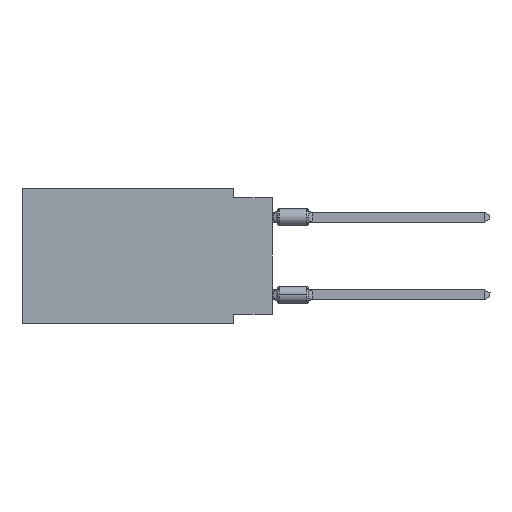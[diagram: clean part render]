
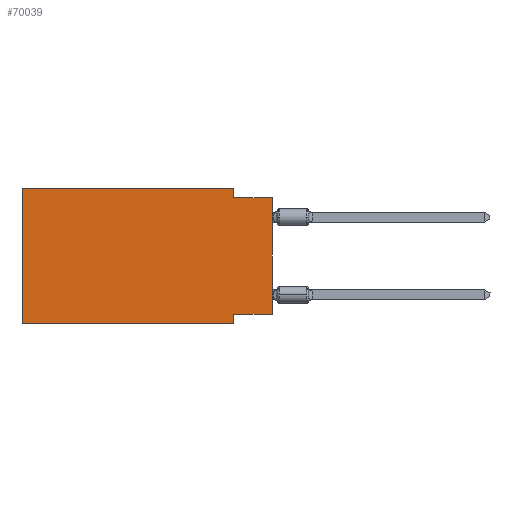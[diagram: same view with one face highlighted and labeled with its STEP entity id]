
A CAD part, left-side view. The second image highlights one B-rep face of the part: STEP entity #70039.
In plain terms, the highlighted planar face has unit normal (-1, 0, 0).
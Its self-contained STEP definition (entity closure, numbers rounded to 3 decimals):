
#1227 = ORIENTED_EDGE ( 'NONE', *, *, #39790, .F. ) ;
#2309 = EDGE_LOOP ( 'NONE', ( #7311, #1227, #25626, #28948, #22406, #39663, #37790, #55043 ) ) ;
#2848 = DIRECTION ( 'NONE',  ( 0., 0., -1. ) ) ;
#3873 = CARTESIAN_POINT ( 'NONE',  ( 0., 16.383, 0. ) ) ;
#4240 = CARTESIAN_POINT ( 'NONE',  ( 0., 16.383, 0. ) ) ;
#4320 = CARTESIAN_POINT ( 'NONE',  ( 0., 2.54, -8.255 ) ) ;
#4486 = VERTEX_POINT ( 'NONE', #47681 ) ;
#7311 = ORIENTED_EDGE ( 'NONE', *, *, #52793, .T. ) ;
#8600 = DIRECTION ( 'NONE',  ( 0., 0., -1. ) ) ;
#12248 = VERTEX_POINT ( 'NONE', #57876 ) ;
#12570 = EDGE_CURVE ( 'NONE', #12248, #4486, #19305, .T. ) ;
#13550 = AXIS2_PLACEMENT_3D ( 'NONE', #3873, #14925, #25629 ) ;
#14925 = DIRECTION ( 'NONE',  ( 1., 0., 0. ) ) ;
#16341 = CARTESIAN_POINT ( 'NONE',  ( 0., 16.383, -8.89 ) ) ;
#18256 = CARTESIAN_POINT ( 'NONE',  ( 0., 2.54, 0. ) ) ;
#19305 = LINE ( 'NONE', #18256, #48768 ) ;
#20276 = VECTOR ( 'NONE', #40275, 1000. ) ;
#22406 = ORIENTED_EDGE ( 'NONE', *, *, #34419, .F. ) ;
#23766 = EDGE_CURVE ( 'NONE', #64450, #54979, #24576, .T. ) ;
#24576 = LINE ( 'NONE', #68429, #20276 ) ;
#25626 = ORIENTED_EDGE ( 'NONE', *, *, #12570, .F. ) ;
#25629 = DIRECTION ( 'NONE',  ( 0., 0., -1. ) ) ;
#26002 = EDGE_CURVE ( 'NONE', #45924, #51246, #53262, .T. ) ;
#26425 = DIRECTION ( 'NONE',  ( 0., 0., 1. ) ) ;
#28948 = ORIENTED_EDGE ( 'NONE', *, *, #46018, .F. ) ;
#29203 = CARTESIAN_POINT ( 'NONE',  ( 0., 0., -0.635 ) ) ;
#31385 = LINE ( 'NONE', #41005, #66672 ) ;
#33119 = CARTESIAN_POINT ( 'NONE',  ( 0., 0., -0.635 ) ) ;
#34211 = CARTESIAN_POINT ( 'NONE',  ( 0., 2.54, -8.89 ) ) ;
#34419 = EDGE_CURVE ( 'NONE', #64450, #67471, #42133, .T. ) ;
#35629 = PLANE ( 'NONE',  #13550 ) ;
#37790 = ORIENTED_EDGE ( 'NONE', *, *, #50009, .F. ) ;
#39663 = ORIENTED_EDGE ( 'NONE', *, *, #23766, .T. ) ;
#39790 = EDGE_CURVE ( 'NONE', #4486, #60204, #50594, .T. ) ;
#40275 = DIRECTION ( 'NONE',  ( 0., -1., 0. ) ) ;
#40370 = LINE ( 'NONE', #4240, #56119 ) ;
#40599 = FACE_OUTER_BOUND ( 'NONE', #2309, .T. ) ;
#41005 = CARTESIAN_POINT ( 'NONE',  ( 0., 2.54, -8.89 ) ) ;
#41175 = CARTESIAN_POINT ( 'NONE',  ( 0., 0., 0. ) ) ;
#42133 = LINE ( 'NONE', #69567, #55509 ) ;
#42575 = VECTOR ( 'NONE', #45591, 1000. ) ;
#42921 = CARTESIAN_POINT ( 'NONE',  ( 0., 0., -8.255 ) ) ;
#45591 = DIRECTION ( 'NONE',  ( 0., -1., 0. ) ) ;
#45924 = VERTEX_POINT ( 'NONE', #65002 ) ;
#46018 = EDGE_CURVE ( 'NONE', #67471, #12248, #40370, .T. ) ;
#47217 = DIRECTION ( 'NONE',  ( 0., 0., 1. ) ) ;
#47681 = CARTESIAN_POINT ( 'NONE',  ( 0., 2.54, -0.635 ) ) ;
#48768 = VECTOR ( 'NONE', #8600, 1000. ) ;
#50009 = EDGE_CURVE ( 'NONE', #51246, #54979, #31385, .T. ) ;
#50594 = LINE ( 'NONE', #29203, #42575 ) ;
#51246 = VERTEX_POINT ( 'NONE', #4320 ) ;
#52793 = EDGE_CURVE ( 'NONE', #45924, #60204, #69679, .T. ) ;
#53262 = LINE ( 'NONE', #42921, #69262 ) ;
#53970 = DIRECTION ( 'NONE',  ( 0., 1., 0. ) ) ;
#54979 = VERTEX_POINT ( 'NONE', #34211 ) ;
#55043 = ORIENTED_EDGE ( 'NONE', *, *, #26002, .F. ) ;
#55509 = VECTOR ( 'NONE', #26425, 1000. ) ;
#56119 = VECTOR ( 'NONE', #58086, 1000. ) ;
#57876 = CARTESIAN_POINT ( 'NONE',  ( 0., 2.54, 0. ) ) ;
#58086 = DIRECTION ( 'NONE',  ( 0., -1., 0. ) ) ;
#60204 = VERTEX_POINT ( 'NONE', #33119 ) ;
#61182 = CARTESIAN_POINT ( 'NONE',  ( 0., 16.383, 0. ) ) ;
#64123 = VECTOR ( 'NONE', #47217, 1000. ) ;
#64450 = VERTEX_POINT ( 'NONE', #16341 ) ;
#65002 = CARTESIAN_POINT ( 'NONE',  ( 0., 0., -8.255 ) ) ;
#66672 = VECTOR ( 'NONE', #2848, 1000. ) ;
#67471 = VERTEX_POINT ( 'NONE', #61182 ) ;
#68429 = CARTESIAN_POINT ( 'NONE',  ( 0., 16.383, -8.89 ) ) ;
#69262 = VECTOR ( 'NONE', #53970, 1000. ) ;
#69567 = CARTESIAN_POINT ( 'NONE',  ( 0., 16.383, 0. ) ) ;
#69679 = LINE ( 'NONE', #41175, #64123 ) ;
#70039 = ADVANCED_FACE ( 'NONE', ( #40599 ), #35629, .F. ) ;
